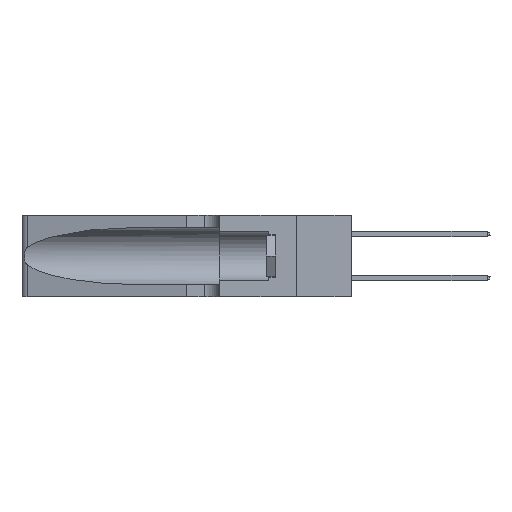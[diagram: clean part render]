
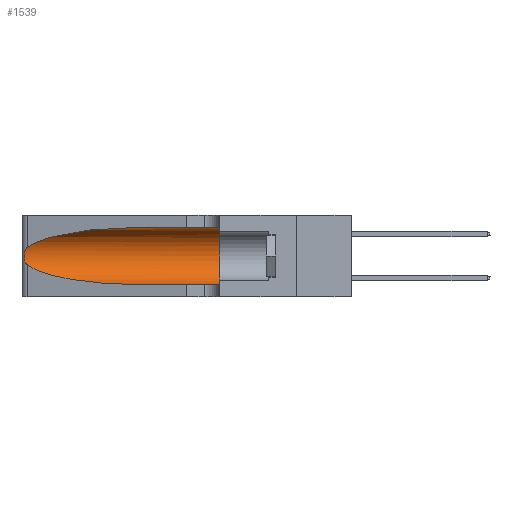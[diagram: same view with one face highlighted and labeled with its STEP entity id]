
A CAD part, left-side view. The second image highlights one B-rep face of the part: STEP entity #1539.
In plain terms, the highlighted cylindrical face has radius 3.308 mm (diameter 6.617 mm), a partial arc.
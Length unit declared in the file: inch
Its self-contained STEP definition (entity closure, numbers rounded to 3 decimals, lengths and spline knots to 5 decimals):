
#796 = CARTESIAN_POINT ( 'NONE',  ( 0.25487, 1.22718, 0.14631 ) ) ;
#1164 = DIRECTION ( 'NONE',  ( 0., -1., 0. ) ) ;
#1539 = ADVANCED_FACE ( 'NONE', ( #10445 ), #15100, .F. ) ;
#1572 = CARTESIAN_POINT ( 'NONE',  ( 0.18966, 0.96281, 0.31525 ) ) ;
#1984 = CARTESIAN_POINT ( 'NONE',  ( 0.2373, 1.15595, 0.08982 ) ) ;
#2580 = ORIENTED_EDGE ( 'NONE', *, *, #7457, .F. ) ;
#3655 = CARTESIAN_POINT ( 'NONE',  ( 0.2373, 1.15595, 0.28018 ) ) ;
#3840 = CARTESIAN_POINT ( 'NONE',  ( 0.25787, 1.23484, 0.2124 ) ) ;
#4071 = CARTESIAN_POINT ( 'NONE',  ( 0.1305, 0.72297, 0.05475 ) ) ;
#4180 = VERTEX_POINT ( 'NONE', #796 ) ;
#4903 =( BOUNDED_CURVE ( )  B_SPLINE_CURVE ( 3, ( #23588, #1572, #3655, #17682 ),
 .UNSPECIFIED., .F., .T. ) 
 B_SPLINE_CURVE_WITH_KNOTS ( ( 4, 4 ),
 ( 1.5708, 2.84003 ),
 .UNSPECIFIED. ) 
 CURVE ( )  GEOMETRIC_REPRESENTATION_ITEM ( )  RATIONAL_B_SPLINE_CURVE ( ( 1., 0.87, 0.87, 1. ) ) 
 REPRESENTATION_ITEM ( '' )  );
#4909 = AXIS2_PLACEMENT_3D ( 'NONE', #10392, #8481, #21987 ) ;
#5895 = CARTESIAN_POINT ( 'NONE',  ( 0.26018, 1.23835, 0.19895 ) ) ;
#6175 = VERTEX_POINT ( 'NONE', #7297 ) ;
#7297 = CARTESIAN_POINT ( 'NONE',  ( 0.1305, 0.35, 0.05475 ) ) ;
#7457 = EDGE_CURVE ( 'NONE', #24615, #6175, #15790, .T. ) ;
#7951 = CARTESIAN_POINT ( 'NONE',  ( 0.26075, 1.23896, 0.178 ) ) ;
#8481 = DIRECTION ( 'NONE',  ( 0., -1., 0. ) ) ;
#9065 = VECTOR ( 'NONE', #1164, 39.37008 ) ;
#9289 = CARTESIAN_POINT ( 'NONE',  ( 0.1305, 0.72297, 0.31525 ) ) ;
#9493 = DIRECTION ( 'NONE',  ( 0., 1., 0. ) ) ;
#9690 = LINE ( 'NONE', #17300, #9065 ) ;
#9953 = CARTESIAN_POINT ( 'NONE',  ( 0.25856, 1.23593, 0.16098 ) ) ;
#10392 = CARTESIAN_POINT ( 'NONE',  ( 0.1305, 1.61858, 0.185 ) ) ;
#10407 = EDGE_CURVE ( 'NONE', #4180, #23790, #20777, .T. ) ;
#10445 = FACE_OUTER_BOUND ( 'NONE', #21947, .T. ) ;
#11418 = ORIENTED_EDGE ( 'NONE', *, *, #10407, .T. ) ;
#11741 = ORIENTED_EDGE ( 'NONE', *, *, #17963, .F. ) ;
#11859 = CARTESIAN_POINT ( 'NONE',  ( 0.25555, 1.22994, 0.2215 ) ) ;
#11940 = CARTESIAN_POINT ( 'NONE',  ( 0.25639, 1.23186, 0.15144 ) ) ;
#13948 = CARTESIAN_POINT ( 'NONE',  ( 0.25487, 1.22718, 0.14631 ) ) ;
#14172 = CARTESIAN_POINT ( 'NONE',  ( 0.25487, 1.22718, 0.22369 ) ) ;
#14983 = EDGE_CURVE ( 'NONE', #19593, #4180, #16143, .T. ) ;
#15100 = CYLINDRICAL_SURFACE ( 'NONE', #4909, 0.13025 ) ;
#15424 = EDGE_CURVE ( 'NONE', #23790, #6175, #9690, .T. ) ;
#15790 = CIRCLE ( 'NONE', #24849, 0.13025 ) ;
#15853 = CARTESIAN_POINT ( 'NONE',  ( 0.25639, 1.23184, 0.21858 ) ) ;
#16090 = CARTESIAN_POINT ( 'NONE',  ( 0.18966, 0.96281, 0.05475 ) ) ;
#16143 = B_SPLINE_CURVE_WITH_KNOTS ( 'NONE', 3,
 ( #25656, #11859, #15853, #3840, #17849, #5895, #19849, #7951, #21856, #9953, #23845, #11940, #25833, #13948 ),
 .UNSPECIFIED., .F., .F.,
 ( 4, 2, 2, 2, 2, 2, 4 ),
 ( 0., 0.00027, 0.00053, 0.00107, 0.0016, 0.00187, 0.00214 ),
 .UNSPECIFIED. ) ;
#17300 = CARTESIAN_POINT ( 'NONE',  ( 0.1305, 1.61858, 0.05475 ) ) ;
#17329 = ORIENTED_EDGE ( 'NONE', *, *, #15424, .T. ) ;
#17682 = CARTESIAN_POINT ( 'NONE',  ( 0.25487, 1.22718, 0.22369 ) ) ;
#17849 = CARTESIAN_POINT ( 'NONE',  ( 0.25854, 1.2359, 0.20912 ) ) ;
#17963 = EDGE_CURVE ( 'NONE', #17989, #24615, #23978, .T. ) ;
#17989 = VERTEX_POINT ( 'NONE', #9289 ) ;
#19593 = VERTEX_POINT ( 'NONE', #14172 ) ;
#19849 = CARTESIAN_POINT ( 'NONE',  ( 0.26075, 1.23896, 0.19203 ) ) ;
#20537 = CARTESIAN_POINT ( 'NONE',  ( 0.1305, 0.35, 0.31525 ) ) ;
#20777 =( BOUNDED_CURVE ( )  B_SPLINE_CURVE ( 3, ( #25975, #1984, #16090, #4071 ),
 .UNSPECIFIED., .F., .F. ) 
 B_SPLINE_CURVE_WITH_KNOTS ( ( 4, 4 ),
 ( 3.44316, 4.71239 ),
 .UNSPECIFIED. ) 
 CURVE ( )  GEOMETRIC_REPRESENTATION_ITEM ( )  RATIONAL_B_SPLINE_CURVE ( ( 1., 0.87, 0.87, 1. ) ) 
 REPRESENTATION_ITEM ( '' )  );
#21230 = CARTESIAN_POINT ( 'NONE',  ( 0.1305, 0.72297, 0.05475 ) ) ;
#21357 = ORIENTED_EDGE ( 'NONE', *, *, #23207, .T. ) ;
#21403 = CARTESIAN_POINT ( 'NONE',  ( 0.1305, 0.35, 0.185 ) ) ;
#21856 = CARTESIAN_POINT ( 'NONE',  ( 0.26017, 1.23833, 0.17102 ) ) ;
#21947 = EDGE_LOOP ( 'NONE', ( #21357, #22916, #11418, #17329, #2580, #11741 ) ) ;
#21987 = DIRECTION ( 'NONE',  ( 0., 0., -1. ) ) ;
#22916 = ORIENTED_EDGE ( 'NONE', *, *, #14983, .T. ) ;
#23096 = CARTESIAN_POINT ( 'NONE',  ( 0.1305, 1.61858, 0.31525 ) ) ;
#23207 = EDGE_CURVE ( 'NONE', #17989, #19593, #4903, .T. ) ;
#23347 = VECTOR ( 'NONE', #25083, 39.37008 ) ;
#23378 = DIRECTION ( 'NONE',  ( 0., 0., 1. ) ) ;
#23588 = CARTESIAN_POINT ( 'NONE',  ( 0.1305, 0.72297, 0.31525 ) ) ;
#23790 = VERTEX_POINT ( 'NONE', #21230 ) ;
#23845 = CARTESIAN_POINT ( 'NONE',  ( 0.25789, 1.23486, 0.15765 ) ) ;
#23978 = LINE ( 'NONE', #23096, #23347 ) ;
#24615 = VERTEX_POINT ( 'NONE', #20537 ) ;
#24849 = AXIS2_PLACEMENT_3D ( 'NONE', #21403, #9493, #23378 ) ;
#25083 = DIRECTION ( 'NONE',  ( 0., -1., 0. ) ) ;
#25656 = CARTESIAN_POINT ( 'NONE',  ( 0.25487, 1.22718, 0.22369 ) ) ;
#25833 = CARTESIAN_POINT ( 'NONE',  ( 0.25555, 1.22993, 0.14849 ) ) ;
#25975 = CARTESIAN_POINT ( 'NONE',  ( 0.25487, 1.22718, 0.14631 ) ) ;
